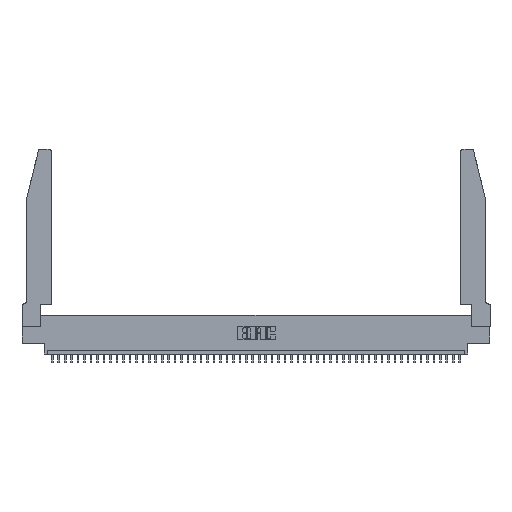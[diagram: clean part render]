
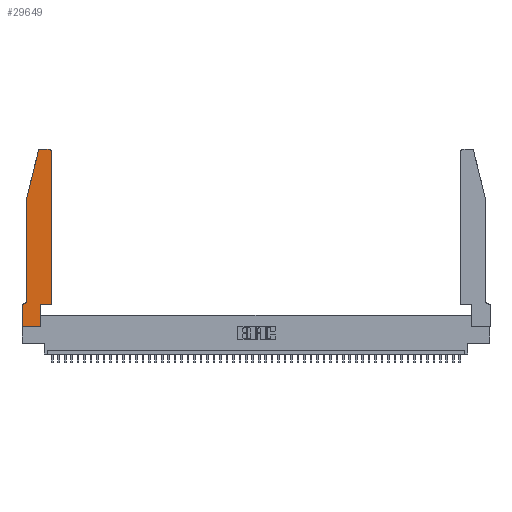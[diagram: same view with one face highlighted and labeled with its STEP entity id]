
A CAD part, top view. The second image highlights one B-rep face of the part: STEP entity #29649.
In plain terms, the highlighted planar face has unit normal (0, 0, 1).
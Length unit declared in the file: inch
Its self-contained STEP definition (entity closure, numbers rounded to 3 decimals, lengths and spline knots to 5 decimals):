
#182 = VERTEX_POINT ( 'NONE', #31528 ) ;
#617 = CIRCLE ( 'NONE', #32585, 0.07 ) ;
#1151 = CARTESIAN_POINT ( 'NONE',  ( 0.4505, 2.72, 0.37 ) ) ;
#1977 = VECTOR ( 'NONE', #41210, 39.37008 ) ;
#1985 = CARTESIAN_POINT ( 'NONE',  ( 0.0755, 2., 0.37 ) ) ;
#2292 = CARTESIAN_POINT ( 'NONE',  ( 0., 0.35, 0.37 ) ) ;
#2504 = LINE ( 'NONE', #5186, #9191 ) ;
#2982 = FACE_OUTER_BOUND ( 'NONE', #19088, .T. ) ;
#4916 = AXIS2_PLACEMENT_3D ( 'NONE', #47677, #24218, #28109 ) ;
#5186 = CARTESIAN_POINT ( 'NONE',  ( 0.0755, 0.35, 0.37 ) ) ;
#5450 = CARTESIAN_POINT ( 'NONE',  ( 0.0755, 0.42, 0.37 ) ) ;
#6043 = CARTESIAN_POINT ( 'NONE',  ( 0.4505, 0.35, 0.37 ) ) ;
#6723 = CARTESIAN_POINT ( 'NONE',  ( 0., 0., 0.37 ) ) ;
#7526 = EDGE_CURVE ( 'NONE', #21724, #29980, #617, .T. ) ;
#7747 = LINE ( 'NONE', #43958, #27711 ) ;
#9191 = VECTOR ( 'NONE', #47965, 39.37008 ) ;
#9576 = CARTESIAN_POINT ( 'NONE',  ( 0.2605, 2.75, 0.37 ) ) ;
#10862 = ORIENTED_EDGE ( 'NONE', *, *, #46327, .T. ) ;
#11752 = CARTESIAN_POINT ( 'NONE',  ( 0.0055, 0.35, 0.37 ) ) ;
#12027 = CIRCLE ( 'NONE', #39461, 0.03 ) ;
#12381 = LINE ( 'NONE', #41591, #13529 ) ;
#12437 = EDGE_CURVE ( 'NONE', #32839, #40335, #12027, .T. ) ;
#13074 = PLANE ( 'NONE',  #27634 ) ;
#13529 = VECTOR ( 'NONE', #30102, 39.37008 ) ;
#13826 = CARTESIAN_POINT ( 'NONE',  ( 0., 0., 0.37 ) ) ;
#13912 = CARTESIAN_POINT ( 'NONE',  ( 0.0755, 2., 0.37 ) ) ;
#14790 = ORIENTED_EDGE ( 'NONE', *, *, #30564, .T. ) ;
#15524 = EDGE_CURVE ( 'NONE', #29075, #42512, #38436, .T. ) ;
#15549 = VECTOR ( 'NONE', #29044, 39.37008 ) ;
#15911 = ORIENTED_EDGE ( 'NONE', *, *, #7526, .T. ) ;
#16223 = CIRCLE ( 'NONE', #4916, 0.03 ) ;
#17853 = CARTESIAN_POINT ( 'NONE',  ( 0.284, 2.75, 0.37 ) ) ;
#18766 = CARTESIAN_POINT ( 'NONE',  ( 0.4505, 0.35, 0.37 ) ) ;
#19088 = EDGE_LOOP ( 'NONE', ( #35545, #46979, #48399, #14790, #15911, #25790, #46420, #46305, #49901, #10862, #28470, #42300 ) ) ;
#19299 = LINE ( 'NONE', #24734, #44642 ) ;
#19407 = EDGE_CURVE ( 'NONE', #40335, #34236, #31647, .T. ) ;
#20250 = VERTEX_POINT ( 'NONE', #6043 ) ;
#21236 = CARTESIAN_POINT ( 'NONE',  ( 0.2865, 0., 0.37 ) ) ;
#21724 = VERTEX_POINT ( 'NONE', #5450 ) ;
#23073 = VECTOR ( 'NONE', #36595, 39.37008 ) ;
#23275 = VECTOR ( 'NONE', #23995, 39.37008 ) ;
#23995 = DIRECTION ( 'NONE',  ( 0., 1., 0. ) ) ;
#24218 = DIRECTION ( 'NONE',  ( 0., 0., 1. ) ) ;
#24435 = LINE ( 'NONE', #18766, #1977 ) ;
#24734 = CARTESIAN_POINT ( 'NONE',  ( 0.0755, 2., 0.37 ) ) ;
#24759 = EDGE_CURVE ( 'NONE', #182, #32839, #40534, .T. ) ;
#24774 = CARTESIAN_POINT ( 'NONE',  ( 0., 0.35, 0.37 ) ) ;
#25790 = ORIENTED_EDGE ( 'NONE', *, *, #47268, .T. ) ;
#26864 = EDGE_CURVE ( 'NONE', #48444, #45473, #30661, .T. ) ;
#27634 = AXIS2_PLACEMENT_3D ( 'NONE', #24774, #40465, #48734 ) ;
#27711 = VECTOR ( 'NONE', #35648, 39.37008 ) ;
#28109 = DIRECTION ( 'NONE',  ( 1., 0., 0. ) ) ;
#28470 = ORIENTED_EDGE ( 'NONE', *, *, #45742, .T. ) ;
#29044 = DIRECTION ( 'NONE',  ( 0., -1., 0. ) ) ;
#29075 = VERTEX_POINT ( 'NONE', #21236 ) ;
#29262 = DIRECTION ( 'NONE',  ( 0., 0., -1. ) ) ;
#29649 = ADVANCED_FACE ( 'NONE', ( #2982 ), #13074, .T. ) ;
#29980 = VERTEX_POINT ( 'NONE', #11752 ) ;
#30102 = DIRECTION ( 'NONE',  ( 0., 1., 0. ) ) ;
#30511 = EDGE_CURVE ( 'NONE', #45473, #29075, #7747, .T. ) ;
#30564 = EDGE_CURVE ( 'NONE', #34236, #21724, #19299, .T. ) ;
#30582 = EDGE_CURVE ( 'NONE', #39442, #182, #16223, .T. ) ;
#30661 = LINE ( 'NONE', #13826, #15549 ) ;
#31528 = CARTESIAN_POINT ( 'NONE',  ( 0.4205, 2.75, 0.37 ) ) ;
#31647 = LINE ( 'NONE', #13912, #36516 ) ;
#32152 = CARTESIAN_POINT ( 'NONE',  ( 0.25487, 2.72718, 0.37 ) ) ;
#32585 = AXIS2_PLACEMENT_3D ( 'NONE', #47520, #29262, #47544 ) ;
#32839 = VERTEX_POINT ( 'NONE', #17853 ) ;
#33141 = CARTESIAN_POINT ( 'NONE',  ( 0.2865, 0.35, 0.37 ) ) ;
#33197 = CARTESIAN_POINT ( 'NONE',  ( 0.284, 2.72, 0.37 ) ) ;
#34236 = VERTEX_POINT ( 'NONE', #1985 ) ;
#35545 = ORIENTED_EDGE ( 'NONE', *, *, #24759, .T. ) ;
#35648 = DIRECTION ( 'NONE',  ( 1., 0., 0. ) ) ;
#36516 = VECTOR ( 'NONE', #40609, 39.37008 ) ;
#36595 = DIRECTION ( 'NONE',  ( -1., 0., 0. ) ) ;
#37616 = DIRECTION ( 'NONE',  ( 0., 0., 1. ) ) ;
#38436 = LINE ( 'NONE', #46962, #23275 ) ;
#39442 = VERTEX_POINT ( 'NONE', #1151 ) ;
#39461 = AXIS2_PLACEMENT_3D ( 'NONE', #33197, #37616, #45243 ) ;
#40335 = VERTEX_POINT ( 'NONE', #32152 ) ;
#40465 = DIRECTION ( 'NONE',  ( 0., 0., 1. ) ) ;
#40534 = LINE ( 'NONE', #9576, #23073 ) ;
#40609 = DIRECTION ( 'NONE',  ( -0.239, -0.971, 0. ) ) ;
#41210 = DIRECTION ( 'NONE',  ( 1., 0., 0. ) ) ;
#41591 = CARTESIAN_POINT ( 'NONE',  ( 0.4505, 0.35, 0.37 ) ) ;
#42300 = ORIENTED_EDGE ( 'NONE', *, *, #30582, .T. ) ;
#42512 = VERTEX_POINT ( 'NONE', #33141 ) ;
#43273 = DIRECTION ( 'NONE',  ( 0., -1., 0. ) ) ;
#43958 = CARTESIAN_POINT ( 'NONE',  ( 0., 0., 0.37 ) ) ;
#44642 = VECTOR ( 'NONE', #43273, 39.37008 ) ;
#45243 = DIRECTION ( 'NONE',  ( 1., 0., 0. ) ) ;
#45473 = VERTEX_POINT ( 'NONE', #6723 ) ;
#45742 = EDGE_CURVE ( 'NONE', #20250, #39442, #12381, .T. ) ;
#46305 = ORIENTED_EDGE ( 'NONE', *, *, #30511, .T. ) ;
#46327 = EDGE_CURVE ( 'NONE', #42512, #20250, #24435, .T. ) ;
#46420 = ORIENTED_EDGE ( 'NONE', *, *, #26864, .T. ) ;
#46962 = CARTESIAN_POINT ( 'NONE',  ( 0.2865, 0.35, 0.37 ) ) ;
#46979 = ORIENTED_EDGE ( 'NONE', *, *, #12437, .T. ) ;
#47268 = EDGE_CURVE ( 'NONE', #29980, #48444, #2504, .T. ) ;
#47520 = CARTESIAN_POINT ( 'NONE',  ( 0.0055, 0.42, 0.37 ) ) ;
#47544 = DIRECTION ( 'NONE',  ( -1., 0., 0. ) ) ;
#47677 = CARTESIAN_POINT ( 'NONE',  ( 0.4205, 2.72, 0.37 ) ) ;
#47965 = DIRECTION ( 'NONE',  ( -1., 0., 0. ) ) ;
#48399 = ORIENTED_EDGE ( 'NONE', *, *, #19407, .T. ) ;
#48444 = VERTEX_POINT ( 'NONE', #2292 ) ;
#48734 = DIRECTION ( 'NONE',  ( 1., 0., 0. ) ) ;
#49901 = ORIENTED_EDGE ( 'NONE', *, *, #15524, .T. ) ;
